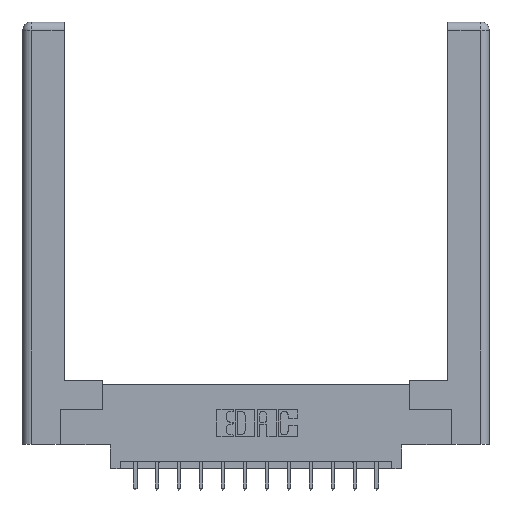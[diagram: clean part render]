
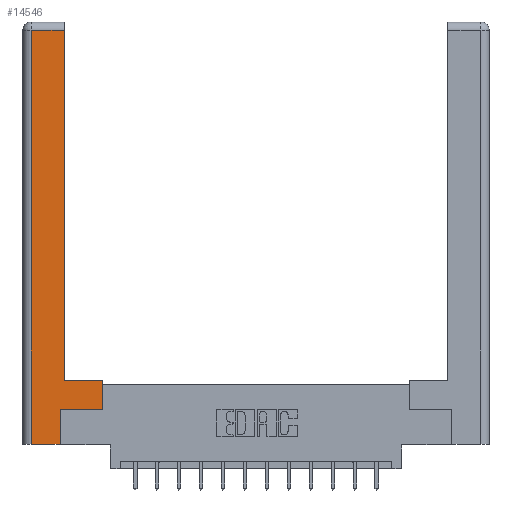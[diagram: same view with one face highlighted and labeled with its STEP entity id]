
A CAD part, top view. The second image highlights one B-rep face of the part: STEP entity #14546.
In plain terms, the highlighted planar face has unit normal (0, 0, 1).
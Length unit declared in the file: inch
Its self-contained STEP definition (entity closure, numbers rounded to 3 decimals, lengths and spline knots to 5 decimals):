
#285 = EDGE_CURVE ( 'NONE', #14368, #8634, #9719, .T. ) ;
#456 = DIRECTION ( 'NONE',  ( -1., 0., 0. ) ) ;
#651 = VECTOR ( 'NONE', #13225, 39.37008 ) ;
#826 = LINE ( 'NONE', #11971, #13596 ) ;
#924 = DIRECTION ( 'NONE',  ( 1., 0., 0. ) ) ;
#1073 = CARTESIAN_POINT ( 'NONE',  ( 0., 0., 0. ) ) ;
#1261 = ORIENTED_EDGE ( 'NONE', *, *, #1562, .T. ) ;
#1485 = ORIENTED_EDGE ( 'NONE', *, *, #14367, .T. ) ;
#1562 = EDGE_CURVE ( 'NONE', #6006, #3158, #12181, .T. ) ;
#1598 = CARTESIAN_POINT ( 'NONE',  ( 0.295, 0.45, 0. ) ) ;
#2087 = CARTESIAN_POINT ( 'NONE',  ( 0.565, 0.45, 0. ) ) ;
#2156 = DIRECTION ( 'NONE',  ( -1., 0., 0. ) ) ;
#2169 = VECTOR ( 'NONE', #5748, 39.37008 ) ;
#2968 = LINE ( 'NONE', #13104, #2169 ) ;
#3133 = VECTOR ( 'NONE', #15910, 39.37008 ) ;
#3158 = VERTEX_POINT ( 'NONE', #1598 ) ;
#3278 = LINE ( 'NONE', #8143, #3880 ) ;
#3294 = CARTESIAN_POINT ( 'NONE',  ( 0.265, 0., 0. ) ) ;
#3354 = FACE_OUTER_BOUND ( 'NONE', #14988, .T. ) ;
#3679 = VECTOR ( 'NONE', #9591, 39.37008 ) ;
#3684 = CARTESIAN_POINT ( 'NONE',  ( 0.0615, 0., 0. ) ) ;
#3880 = VECTOR ( 'NONE', #12956, 39.37008 ) ;
#4218 = CARTESIAN_POINT ( 'NONE',  ( 0.0615, 0., 0. ) ) ;
#4638 = CARTESIAN_POINT ( 'NONE',  ( 0.565, 0.245, 0. ) ) ;
#4770 = ORIENTED_EDGE ( 'NONE', *, *, #9829, .T. ) ;
#4887 = LINE ( 'NONE', #3684, #3133 ) ;
#4919 = ORIENTED_EDGE ( 'NONE', *, *, #10033, .T. ) ;
#5745 = DIRECTION ( 'NONE',  ( 0., 1., 0. ) ) ;
#5748 = DIRECTION ( 'NONE',  ( 0., 1., 0. ) ) ;
#6006 = VERTEX_POINT ( 'NONE', #8584 ) ;
#6191 = AXIS2_PLACEMENT_3D ( 'NONE', #1073, #15915, #2156 ) ;
#6653 = EDGE_CURVE ( 'NONE', #11366, #9953, #3278, .T. ) ;
#6913 = ORIENTED_EDGE ( 'NONE', *, *, #15742, .T. ) ;
#7128 = CARTESIAN_POINT ( 'NONE',  ( 0.295, 0.45, 0. ) ) ;
#7367 = CARTESIAN_POINT ( 'NONE',  ( 0.265, 0.245, 0. ) ) ;
#7851 = VERTEX_POINT ( 'NONE', #7367 ) ;
#8143 = CARTESIAN_POINT ( 'NONE',  ( 0.265, 0., 0. ) ) ;
#8395 = CARTESIAN_POINT ( 'NONE',  ( 0.0615, 2.94, 0. ) ) ;
#8534 = PLANE ( 'NONE',  #6191 ) ;
#8584 = CARTESIAN_POINT ( 'NONE',  ( 0.565, 0.45, 0. ) ) ;
#8634 = VERTEX_POINT ( 'NONE', #8395 ) ;
#9148 = CARTESIAN_POINT ( 'NONE',  ( 0.0615, 2.94, 0. ) ) ;
#9192 = LINE ( 'NONE', #2087, #651 ) ;
#9577 = VERTEX_POINT ( 'NONE', #12643 ) ;
#9591 = DIRECTION ( 'NONE',  ( -1., 0., 0. ) ) ;
#9706 = ORIENTED_EDGE ( 'NONE', *, *, #6653, .T. ) ;
#9719 = LINE ( 'NONE', #9148, #10115 ) ;
#9829 = EDGE_CURVE ( 'NONE', #7851, #9577, #14760, .T. ) ;
#9953 = VERTEX_POINT ( 'NONE', #3294 ) ;
#10033 = EDGE_CURVE ( 'NONE', #9577, #6006, #9192, .T. ) ;
#10115 = VECTOR ( 'NONE', #456, 39.37008 ) ;
#10474 = EDGE_CURVE ( 'NONE', #9953, #7851, #826, .T. ) ;
#11103 = VECTOR ( 'NONE', #924, 39.37008 ) ;
#11366 = VERTEX_POINT ( 'NONE', #4218 ) ;
#11971 = CARTESIAN_POINT ( 'NONE',  ( 0.265, 0.245, 0. ) ) ;
#12181 = LINE ( 'NONE', #7128, #3679 ) ;
#12639 = ORIENTED_EDGE ( 'NONE', *, *, #10474, .T. ) ;
#12643 = CARTESIAN_POINT ( 'NONE',  ( 0.565, 0.245, 0. ) ) ;
#12956 = DIRECTION ( 'NONE',  ( 1., 0., 0. ) ) ;
#13104 = CARTESIAN_POINT ( 'NONE',  ( 0.295, 3., 0. ) ) ;
#13225 = DIRECTION ( 'NONE',  ( 0., 1., 0. ) ) ;
#13596 = VECTOR ( 'NONE', #5745, 39.37008 ) ;
#14163 = ORIENTED_EDGE ( 'NONE', *, *, #285, .T. ) ;
#14367 = EDGE_CURVE ( 'NONE', #3158, #14368, #2968, .T. ) ;
#14368 = VERTEX_POINT ( 'NONE', #15566 ) ;
#14546 = ADVANCED_FACE ( 'NONE', ( #3354 ), #8534, .F. ) ;
#14760 = LINE ( 'NONE', #4638, #11103 ) ;
#14988 = EDGE_LOOP ( 'NONE', ( #1485, #14163, #6913, #9706, #12639, #4770, #4919, #1261 ) ) ;
#15566 = CARTESIAN_POINT ( 'NONE',  ( 0.295, 2.94, 0. ) ) ;
#15742 = EDGE_CURVE ( 'NONE', #8634, #11366, #4887, .T. ) ;
#15910 = DIRECTION ( 'NONE',  ( 0., -1., 0. ) ) ;
#15915 = DIRECTION ( 'NONE',  ( 0., 0., -1. ) ) ;
